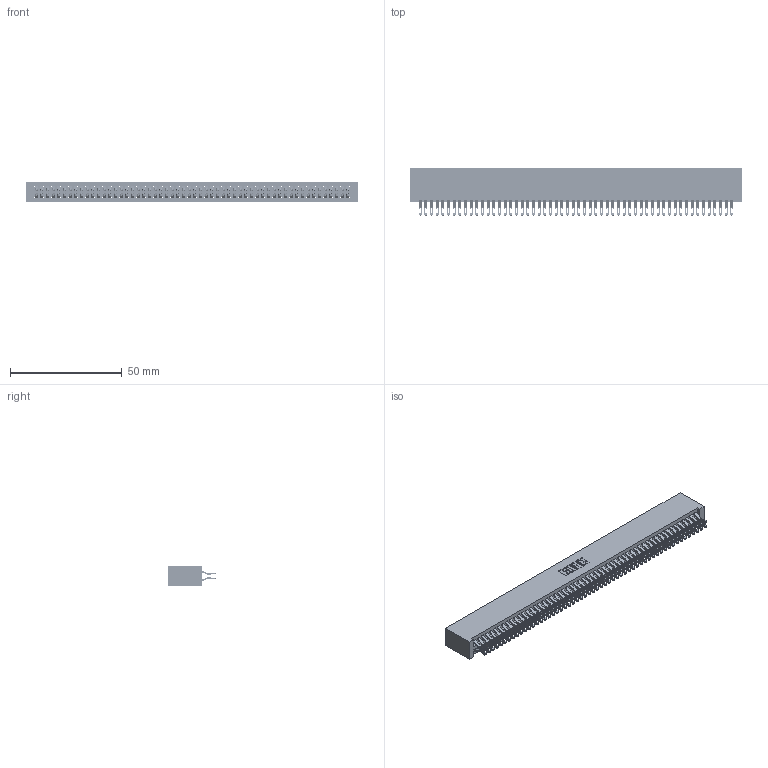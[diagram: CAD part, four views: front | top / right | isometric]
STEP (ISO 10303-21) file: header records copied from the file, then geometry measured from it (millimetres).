
FILE_DESCRIPTION (( 'STEP AP203' ), '1' );
FILE_NAME ('395-112-555-201.STEP', '2019-10-27T15:49:16', ( '' ), ( '' ), 'SwSTEP 2.0', 'SolidWorks 2016', '' );
FILE_SCHEMA (( 'CONFIG_CONTROL_DESIGN' ));
Length unit declared in the file: inch
Products named in the file (3): 395-112-555-201; 345 Part_No Mounting Lugs; 345-292-001_555 Tail
Assembly tree (113 placements, depth 2):
  395-112-555-201
    345 Part_No Mounting Lugs
    345-292-001_555 Tail  x112
Bounding box: 148.84 x 21.13 x 9.4 mm (x, y, z)
Volume: 15529.6 mm3; surface area: 24659.7 mm2
Topology: 113 solids, 113 shells, 6390 faces, 20141 edges, 13426 vertices
Faces by surface type: plane 3548, cylinder 2842
Entity records: 42103 total; most frequent: CARTESIAN_POINT 7078, ORIENTED_EDGE 6982, DIRECTION 6187, EDGE_CURVE 3491, VECTOR 3123, LINE 3123, VERTEX_POINT 2326, AXIS2_PLACEMENT_3D 1532
